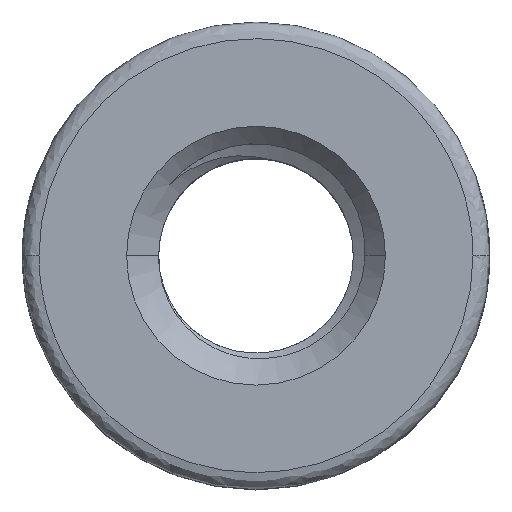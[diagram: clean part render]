
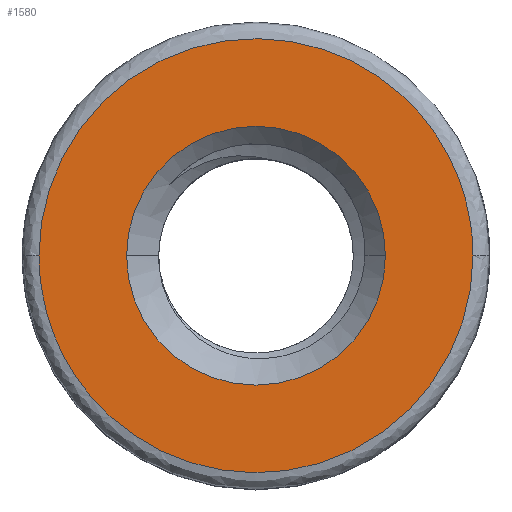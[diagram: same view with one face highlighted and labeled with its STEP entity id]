
A CAD part, top view. The second image highlights one B-rep face of the part: STEP entity #1580.
In plain terms, the highlighted planar face has unit normal (0, 0, 1).
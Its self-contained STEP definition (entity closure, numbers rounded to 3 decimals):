
#30 = PLANE ( 'NONE',  #2609 ) ;
#152 = EDGE_CURVE ( 'NONE', #3432, #2369, #3815, .T. ) ;
#256 = CARTESIAN_POINT ( 'NONE',  ( -5.153, 0., 0. ) ) ;
#312 = DIRECTION ( 'NONE',  ( 0., 0., 1. ) ) ;
#321 = CARTESIAN_POINT ( 'NONE',  ( 5.153, 0., 0. ) ) ;
#482 = CARTESIAN_POINT ( 'NONE',  ( 5.153, 0., 0. ) ) ;
#633 = CARTESIAN_POINT ( 'NONE',  ( 3.073, 0., 0. ) ) ;
#635 = EDGE_CURVE ( 'NONE', #3962, #1714, #4454, .T. ) ;
#902 = ORIENTED_EDGE ( 'NONE', *, *, #152, .F. ) ;
#1058 = DIRECTION ( 'NONE',  ( 1., 0., 0. ) ) ;
#1080 = DIRECTION ( 'NONE',  ( 0., 0., 1. ) ) ;
#1098 = CARTESIAN_POINT ( 'NONE',  ( -5.153, -10.306, 0. ) ) ;
#1099 = CARTESIAN_POINT ( 'NONE',  ( 0., 0., 0. ) ) ;
#1183 = EDGE_LOOP ( 'NONE', ( #3314, #2344 ) ) ;
#1280 = FACE_OUTER_BOUND ( 'NONE', #1767, .T. ) ;
#1580 = ADVANCED_FACE ( 'NONE', ( #1280, #4406 ), #30, .F. ) ;
#1714 = VERTEX_POINT ( 'NONE', #633 ) ;
#1767 = EDGE_LOOP ( 'NONE', ( #902, #5217 ) ) ;
#1928 = CARTESIAN_POINT ( 'NONE',  ( 5.153, -10.306, 0. ) ) ;
#2192 = CARTESIAN_POINT ( 'NONE',  ( -5.153, 10.306, 0. ) ) ;
#2217 = CARTESIAN_POINT ( 'NONE',  ( 0., 3.073, 0. ) ) ;
#2344 = ORIENTED_EDGE ( 'NONE', *, *, #635, .F. ) ;
#2369 = VERTEX_POINT ( 'NONE', #4808 ) ;
#2551 = EDGE_CURVE ( 'NONE', #1714, #3962, #2772, .T. ) ;
#2609 = AXIS2_PLACEMENT_3D ( 'NONE', #2217, #4957, #3067 ) ;
#2663 = CARTESIAN_POINT ( 'NONE',  ( -5.153, 0., 0. ) ) ;
#2730 = EDGE_CURVE ( 'NONE', #2369, #3432, #4783, .T. ) ;
#2772 = CIRCLE ( 'NONE', #3057, 3.073 ) ;
#2859 = CARTESIAN_POINT ( 'NONE',  ( 5.153, 0., 0. ) ) ;
#2937 = CARTESIAN_POINT ( 'NONE',  ( 0., 0., 0. ) ) ;
#3057 = AXIS2_PLACEMENT_3D ( 'NONE', #2937, #312, #3316 ) ;
#3067 = DIRECTION ( 'NONE',  ( -1., 0., 0. ) ) ;
#3074 = CARTESIAN_POINT ( 'NONE',  ( 5.153, 10.306, 0. ) ) ;
#3168 = AXIS2_PLACEMENT_3D ( 'NONE', #1099, #1080, #1058 ) ;
#3291 = CARTESIAN_POINT ( 'NONE',  ( -3.073, 0., 0. ) ) ;
#3314 = ORIENTED_EDGE ( 'NONE', *, *, #2551, .F. ) ;
#3316 = DIRECTION ( 'NONE',  ( 1., 0., 0. ) ) ;
#3432 = VERTEX_POINT ( 'NONE', #2859 ) ;
#3815 =( BOUNDED_CURVE ( )  B_SPLINE_CURVE ( 3, ( #321, #1928, #1098, #256 ),
 .UNSPECIFIED., .F., .F. ) 
 B_SPLINE_CURVE_WITH_KNOTS ( ( 4, 4 ),
 ( 0., 1. ),
 .UNSPECIFIED. ) 
 CURVE ( )  GEOMETRIC_REPRESENTATION_ITEM ( )  RATIONAL_B_SPLINE_CURVE ( ( 1., 0.333, 0.333, 1. ) ) 
 REPRESENTATION_ITEM ( '' )  );
#3962 = VERTEX_POINT ( 'NONE', #3291 ) ;
#4406 = FACE_BOUND ( 'NONE', #1183, .T. ) ;
#4454 = CIRCLE ( 'NONE', #3168, 3.073 ) ;
#4783 =( BOUNDED_CURVE ( )  B_SPLINE_CURVE ( 3, ( #2663, #2192, #3074, #482 ),
 .UNSPECIFIED., .F., .F. ) 
 B_SPLINE_CURVE_WITH_KNOTS ( ( 4, 4 ),
 ( 0., 1. ),
 .UNSPECIFIED. ) 
 CURVE ( )  GEOMETRIC_REPRESENTATION_ITEM ( )  RATIONAL_B_SPLINE_CURVE ( ( 1., 0.333, 0.333, 1. ) ) 
 REPRESENTATION_ITEM ( '' )  );
#4808 = CARTESIAN_POINT ( 'NONE',  ( -5.153, 0., 0. ) ) ;
#4957 = DIRECTION ( 'NONE',  ( 0., 0., -1. ) ) ;
#5217 = ORIENTED_EDGE ( 'NONE', *, *, #2730, .F. ) ;
